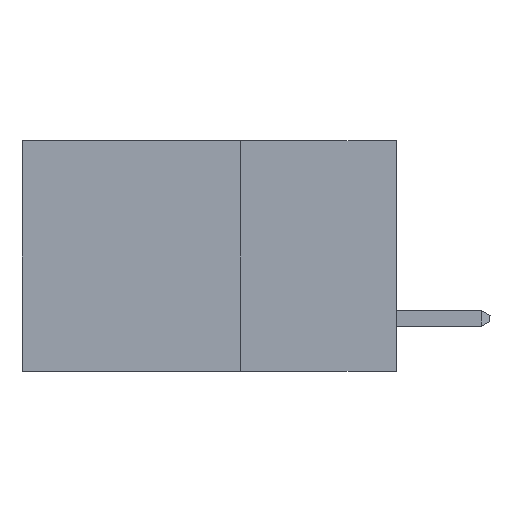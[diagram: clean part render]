
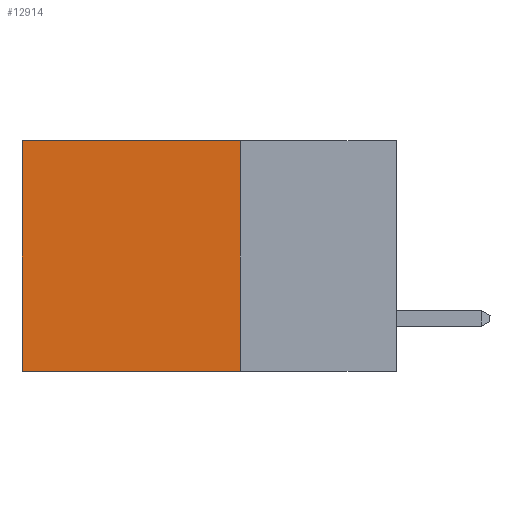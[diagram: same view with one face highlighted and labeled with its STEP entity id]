
A CAD part, left-side view. The second image highlights one B-rep face of the part: STEP entity #12914.
In plain terms, the highlighted planar face has unit normal (-1, 0, 0).
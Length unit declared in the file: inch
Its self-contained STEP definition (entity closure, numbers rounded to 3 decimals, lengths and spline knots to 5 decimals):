
#318 = ORIENTED_EDGE ( 'NONE', *, *, #1002, .T. ) ;
#744 = EDGE_CURVE ( 'NONE', #8279, #12883, #10780, .T. ) ;
#1002 = EDGE_CURVE ( 'NONE', #8279, #2175, #1015, .T. ) ;
#1015 = LINE ( 'NONE', #10905, #6914 ) ;
#1122 = CARTESIAN_POINT ( 'NONE',  ( 0.2615, 0.25, -0.37 ) ) ;
#1286 = DIRECTION ( 'NONE',  ( 0., 1., 0. ) ) ;
#1327 = DIRECTION ( 'NONE',  ( 1., 0., 0. ) ) ;
#1762 = VERTEX_POINT ( 'NONE', #2396 ) ;
#2175 = VERTEX_POINT ( 'NONE', #14287 ) ;
#2396 = CARTESIAN_POINT ( 'NONE',  ( 0.2615, 0.6, -0.37 ) ) ;
#2882 = EDGE_CURVE ( 'NONE', #12883, #1762, #6352, .T. ) ;
#3653 = CARTESIAN_POINT ( 'NONE',  ( 0.2615, 0.25, -0.37 ) ) ;
#4453 = EDGE_LOOP ( 'NONE', ( #10540, #7050, #9723, #318 ) ) ;
#4513 = AXIS2_PLACEMENT_3D ( 'NONE', #3653, #1327, #9465 ) ;
#4686 = DIRECTION ( 'NONE',  ( 0., 0., -1. ) ) ;
#5096 = VECTOR ( 'NONE', #4686, 39.37008 ) ;
#5676 = LINE ( 'NONE', #11897, #8026 ) ;
#6032 = FACE_OUTER_BOUND ( 'NONE', #4453, .T. ) ;
#6352 = LINE ( 'NONE', #1122, #12246 ) ;
#6914 = VECTOR ( 'NONE', #12861, 39.37008 ) ;
#7050 = ORIENTED_EDGE ( 'NONE', *, *, #2882, .F. ) ;
#8026 = VECTOR ( 'NONE', #8604, 39.37008 ) ;
#8279 = VERTEX_POINT ( 'NONE', #11872 ) ;
#8604 = DIRECTION ( 'NONE',  ( 0., 0., -1. ) ) ;
#9465 = DIRECTION ( 'NONE',  ( 0., 0., -1. ) ) ;
#9723 = ORIENTED_EDGE ( 'NONE', *, *, #744, .F. ) ;
#10540 = ORIENTED_EDGE ( 'NONE', *, *, #12527, .T. ) ;
#10780 = LINE ( 'NONE', #11750, #5096 ) ;
#10905 = CARTESIAN_POINT ( 'NONE',  ( 0.2615, 0.25, 0. ) ) ;
#11750 = CARTESIAN_POINT ( 'NONE',  ( 0.2615, 0.25, -0.37 ) ) ;
#11872 = CARTESIAN_POINT ( 'NONE',  ( 0.2615, 0.25, 0. ) ) ;
#11897 = CARTESIAN_POINT ( 'NONE',  ( 0.2615, 0.6, -0.37 ) ) ;
#12246 = VECTOR ( 'NONE', #1286, 39.37008 ) ;
#12527 = EDGE_CURVE ( 'NONE', #2175, #1762, #5676, .T. ) ;
#12612 = CARTESIAN_POINT ( 'NONE',  ( 0.2615, 0.25, -0.37 ) ) ;
#12861 = DIRECTION ( 'NONE',  ( 0., 1., 0. ) ) ;
#12883 = VERTEX_POINT ( 'NONE', #12612 ) ;
#12914 = ADVANCED_FACE ( 'NONE', ( #6032 ), #13753, .F. ) ;
#13753 = PLANE ( 'NONE',  #4513 ) ;
#14287 = CARTESIAN_POINT ( 'NONE',  ( 0.2615, 0.6, 0. ) ) ;
